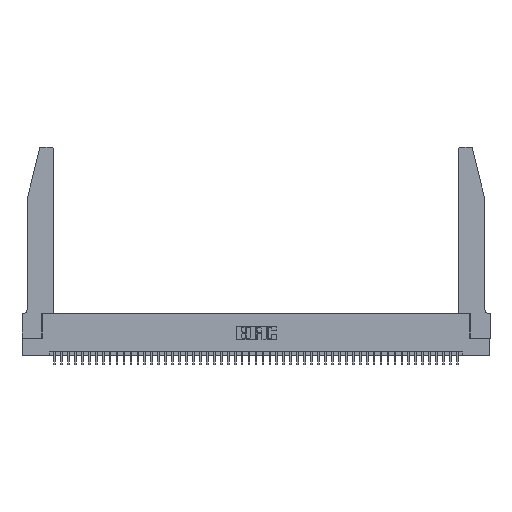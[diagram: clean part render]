
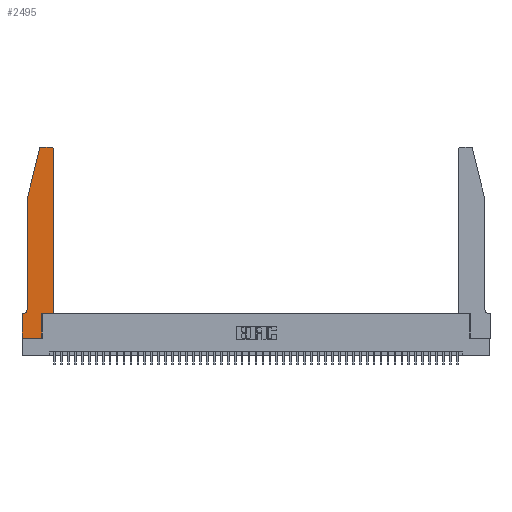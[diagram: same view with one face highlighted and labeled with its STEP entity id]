
A CAD part, top view. The second image highlights one B-rep face of the part: STEP entity #2495.
In plain terms, the highlighted planar face has unit normal (0, 0, 1).
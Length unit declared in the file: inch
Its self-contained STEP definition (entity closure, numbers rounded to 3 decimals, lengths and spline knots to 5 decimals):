
#990 = CARTESIAN_POINT ( 'NONE',  ( 0.0755, 2., 0.37 ) ) ;
#1280 = DIRECTION ( 'NONE',  ( -1., 0., 0. ) ) ;
#1438 = VERTEX_POINT ( 'NONE', #20232 ) ;
#2495 = ADVANCED_FACE ( 'NONE', ( #37981 ), #10904, .T. ) ;
#3049 = LINE ( 'NONE', #7117, #41928 ) ;
#3126 = CARTESIAN_POINT ( 'NONE',  ( 0.0755, 0.35, 0.37 ) ) ;
#3858 = CARTESIAN_POINT ( 'NONE',  ( 0., 0., 0.37 ) ) ;
#4119 = CARTESIAN_POINT ( 'NONE',  ( 0., 0.35, 0.37 ) ) ;
#4333 = DIRECTION ( 'NONE',  ( -1., 0., 0. ) ) ;
#4398 = CIRCLE ( 'NONE', #19895, 0.03 ) ;
#5351 = CARTESIAN_POINT ( 'NONE',  ( 0.4505, 0.35, 0.37 ) ) ;
#6207 = VERTEX_POINT ( 'NONE', #18181 ) ;
#6894 = CARTESIAN_POINT ( 'NONE',  ( 0.4505, 0.35, 0.37 ) ) ;
#6988 = CARTESIAN_POINT ( 'NONE',  ( 0.25487, 2.72718, 0.37 ) ) ;
#7117 = CARTESIAN_POINT ( 'NONE',  ( 0.2865, 0.35, 0.37 ) ) ;
#7266 = LINE ( 'NONE', #5351, #37315 ) ;
#7583 = VECTOR ( 'NONE', #43299, 39.37008 ) ;
#7825 = LINE ( 'NONE', #3858, #17815 ) ;
#9154 = EDGE_CURVE ( 'NONE', #44158, #33892, #4398, .T. ) ;
#10826 = ORIENTED_EDGE ( 'NONE', *, *, #47725, .T. ) ;
#10879 = CARTESIAN_POINT ( 'NONE',  ( 0.284, 2.72, 0.37 ) ) ;
#10904 = PLANE ( 'NONE',  #40254 ) ;
#10996 = EDGE_CURVE ( 'NONE', #43189, #42362, #3049, .T. ) ;
#11151 = CIRCLE ( 'NONE', #27526, 0.03 ) ;
#11638 = EDGE_CURVE ( 'NONE', #32658, #15838, #35970, .T. ) ;
#11741 = ORIENTED_EDGE ( 'NONE', *, *, #10996, .T. ) ;
#12163 = EDGE_CURVE ( 'NONE', #1438, #21718, #11151, .T. ) ;
#12300 = EDGE_CURVE ( 'NONE', #33892, #43339, #37681, .T. ) ;
#12530 = LINE ( 'NONE', #41888, #21346 ) ;
#12820 = ORIENTED_EDGE ( 'NONE', *, *, #12163, .T. ) ;
#13583 = EDGE_CURVE ( 'NONE', #6207, #43189, #31747, .T. ) ;
#13704 = DIRECTION ( 'NONE',  ( 0., 0., 1. ) ) ;
#14650 = DIRECTION ( 'NONE',  ( 1., 0., 0. ) ) ;
#15204 = ORIENTED_EDGE ( 'NONE', *, *, #44434, .T. ) ;
#15838 = VERTEX_POINT ( 'NONE', #4119 ) ;
#17201 = EDGE_CURVE ( 'NONE', #21718, #44158, #12530, .T. ) ;
#17366 = CARTESIAN_POINT ( 'NONE',  ( 0.0755, 2., 0.37 ) ) ;
#17815 = VECTOR ( 'NONE', #45205, 39.37008 ) ;
#18181 = CARTESIAN_POINT ( 'NONE',  ( 0., 0., 0.37 ) ) ;
#18469 = CARTESIAN_POINT ( 'NONE',  ( 0., 0.35, 0.37 ) ) ;
#19119 = CARTESIAN_POINT ( 'NONE',  ( 0.2865, 0., 0.37 ) ) ;
#19582 = ORIENTED_EDGE ( 'NONE', *, *, #9154, .T. ) ;
#19895 = AXIS2_PLACEMENT_3D ( 'NONE', #10879, #37242, #14650 ) ;
#20232 = CARTESIAN_POINT ( 'NONE',  ( 0.4505, 2.72, 0.37 ) ) ;
#20740 = CARTESIAN_POINT ( 'NONE',  ( 0.4505, 0.35, 0.37 ) ) ;
#21346 = VECTOR ( 'NONE', #4333, 39.37008 ) ;
#21718 = VERTEX_POINT ( 'NONE', #44118 ) ;
#21761 = CARTESIAN_POINT ( 'NONE',  ( 0.0755, 2., 0.37 ) ) ;
#21804 = DIRECTION ( 'NONE',  ( 1., 0., 0. ) ) ;
#22268 = DIRECTION ( 'NONE',  ( 1., 0., 0. ) ) ;
#22439 = LINE ( 'NONE', #17366, #33625 ) ;
#23351 = CARTESIAN_POINT ( 'NONE',  ( 0.0755, 0.42, 0.37 ) ) ;
#23843 = DIRECTION ( 'NONE',  ( 0., 0., -1. ) ) ;
#24086 = AXIS2_PLACEMENT_3D ( 'NONE', #46404, #23843, #1280 ) ;
#24110 = ORIENTED_EDGE ( 'NONE', *, *, #29940, .T. ) ;
#24757 = VECTOR ( 'NONE', #25652, 39.37008 ) ;
#25391 = DIRECTION ( 'NONE',  ( -0.239, -0.971, 0. ) ) ;
#25652 = DIRECTION ( 'NONE',  ( -1., 0., 0. ) ) ;
#25772 = CARTESIAN_POINT ( 'NONE',  ( 0.2865, 0.35, 0.37 ) ) ;
#26414 = LINE ( 'NONE', #20740, #7583 ) ;
#26446 = VECTOR ( 'NONE', #25391, 39.37008 ) ;
#27526 = AXIS2_PLACEMENT_3D ( 'NONE', #36286, #13704, #40079 ) ;
#29303 = ORIENTED_EDGE ( 'NONE', *, *, #17201, .T. ) ;
#29360 = CARTESIAN_POINT ( 'NONE',  ( 0., 0., 0.37 ) ) ;
#29940 = EDGE_CURVE ( 'NONE', #35099, #1438, #7266, .T. ) ;
#30126 = CARTESIAN_POINT ( 'NONE',  ( 0.0055, 0.35, 0.37 ) ) ;
#30692 = CIRCLE ( 'NONE', #24086, 0.07 ) ;
#31747 = LINE ( 'NONE', #29360, #40589 ) ;
#31894 = ORIENTED_EDGE ( 'NONE', *, *, #11638, .T. ) ;
#32658 = VERTEX_POINT ( 'NONE', #30126 ) ;
#33625 = VECTOR ( 'NONE', #43905, 39.37008 ) ;
#33892 = VERTEX_POINT ( 'NONE', #6988 ) ;
#35099 = VERTEX_POINT ( 'NONE', #6894 ) ;
#35489 = DIRECTION ( 'NONE',  ( 0., 1., 0. ) ) ;
#35970 = LINE ( 'NONE', #3126, #24757 ) ;
#35985 = CARTESIAN_POINT ( 'NONE',  ( 0.284, 2.75, 0.37 ) ) ;
#36286 = CARTESIAN_POINT ( 'NONE',  ( 0.4205, 2.72, 0.37 ) ) ;
#37242 = DIRECTION ( 'NONE',  ( 0., 0., 1. ) ) ;
#37252 = DIRECTION ( 'NONE',  ( 0., 1., 0. ) ) ;
#37315 = VECTOR ( 'NONE', #35489, 39.37008 ) ;
#37681 = LINE ( 'NONE', #21761, #26446 ) ;
#37815 = EDGE_CURVE ( 'NONE', #42362, #35099, #26414, .T. ) ;
#37981 = FACE_OUTER_BOUND ( 'NONE', #38486, .T. ) ;
#38486 = EDGE_LOOP ( 'NONE', ( #29303, #19582, #43257, #42148, #10826, #31894, #15204, #48499, #11741, #48153, #24110, #12820 ) ) ;
#39525 = VERTEX_POINT ( 'NONE', #23351 ) ;
#40079 = DIRECTION ( 'NONE',  ( 1., 0., 0. ) ) ;
#40254 = AXIS2_PLACEMENT_3D ( 'NONE', #18469, #44848, #22268 ) ;
#40589 = VECTOR ( 'NONE', #21804, 39.37008 ) ;
#41888 = CARTESIAN_POINT ( 'NONE',  ( 0.2605, 2.75, 0.37 ) ) ;
#41928 = VECTOR ( 'NONE', #37252, 39.37008 ) ;
#42148 = ORIENTED_EDGE ( 'NONE', *, *, #47931, .T. ) ;
#42362 = VERTEX_POINT ( 'NONE', #25772 ) ;
#43189 = VERTEX_POINT ( 'NONE', #19119 ) ;
#43257 = ORIENTED_EDGE ( 'NONE', *, *, #12300, .T. ) ;
#43299 = DIRECTION ( 'NONE',  ( 1., 0., 0. ) ) ;
#43339 = VERTEX_POINT ( 'NONE', #990 ) ;
#43905 = DIRECTION ( 'NONE',  ( 0., -1., 0. ) ) ;
#44118 = CARTESIAN_POINT ( 'NONE',  ( 0.4205, 2.75, 0.37 ) ) ;
#44158 = VERTEX_POINT ( 'NONE', #35985 ) ;
#44434 = EDGE_CURVE ( 'NONE', #15838, #6207, #7825, .T. ) ;
#44848 = DIRECTION ( 'NONE',  ( 0., 0., 1. ) ) ;
#45205 = DIRECTION ( 'NONE',  ( 0., -1., 0. ) ) ;
#46404 = CARTESIAN_POINT ( 'NONE',  ( 0.0055, 0.42, 0.37 ) ) ;
#47725 = EDGE_CURVE ( 'NONE', #39525, #32658, #30692, .T. ) ;
#47931 = EDGE_CURVE ( 'NONE', #43339, #39525, #22439, .T. ) ;
#48153 = ORIENTED_EDGE ( 'NONE', *, *, #37815, .T. ) ;
#48499 = ORIENTED_EDGE ( 'NONE', *, *, #13583, .T. ) ;
